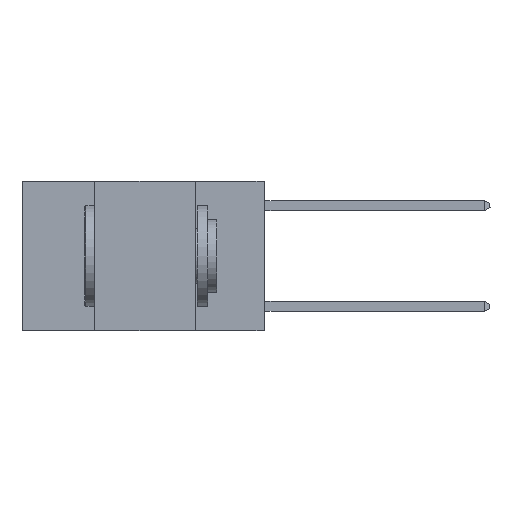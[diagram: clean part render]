
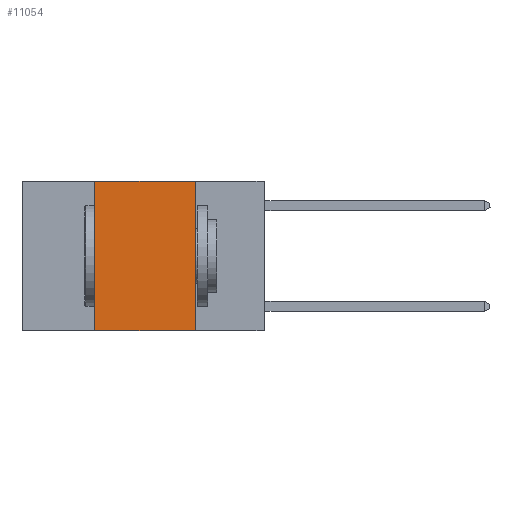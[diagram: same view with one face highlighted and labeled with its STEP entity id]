
A CAD part, left-side view. The second image highlights one B-rep face of the part: STEP entity #11054.
In plain terms, the highlighted planar face has unit normal (-1, 0, 0).
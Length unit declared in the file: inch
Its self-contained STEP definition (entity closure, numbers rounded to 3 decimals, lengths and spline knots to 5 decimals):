
#146 = CARTESIAN_POINT ( 'NONE',  ( 0., 0.6, -0.37 ) ) ;
#241 = VECTOR ( 'NONE', #4468, 39.37008 ) ;
#398 = AXIS2_PLACEMENT_3D ( 'NONE', #4768, #12748, #2808 ) ;
#622 = CARTESIAN_POINT ( 'NONE',  ( 0., 0.6, 0. ) ) ;
#764 = LINE ( 'NONE', #622, #5797 ) ;
#1096 = LINE ( 'NONE', #146, #2507 ) ;
#1280 = CARTESIAN_POINT ( 'NONE',  ( 0., 0.17, 0. ) ) ;
#1683 = CARTESIAN_POINT ( 'NONE',  ( 0., 0.17, 0. ) ) ;
#1985 = ORIENTED_EDGE ( 'NONE', *, *, #12948, .F. ) ;
#2211 = DIRECTION ( 'NONE',  ( 0., -1., 0. ) ) ;
#2241 = CARTESIAN_POINT ( 'NONE',  ( 0., 0.42, 0. ) ) ;
#2301 = CARTESIAN_POINT ( 'NONE',  ( 0., 0.42, 0. ) ) ;
#2507 = VECTOR ( 'NONE', #2211, 39.37008 ) ;
#2808 = DIRECTION ( 'NONE',  ( 0., 0., -1. ) ) ;
#3441 = LINE ( 'NONE', #2241, #241 ) ;
#3780 = CARTESIAN_POINT ( 'NONE',  ( 0., 0.42, -0.37 ) ) ;
#4468 = DIRECTION ( 'NONE',  ( 0., 0., 1. ) ) ;
#4728 = VERTEX_POINT ( 'NONE', #1280 ) ;
#4768 = CARTESIAN_POINT ( 'NONE',  ( 0., 0.6, 0. ) ) ;
#5736 = EDGE_CURVE ( 'NONE', #10228, #8686, #3441, .T. ) ;
#5797 = VECTOR ( 'NONE', #8819, 39.37008 ) ;
#6475 = ORIENTED_EDGE ( 'NONE', *, *, #5736, .F. ) ;
#6896 = FACE_OUTER_BOUND ( 'NONE', #11346, .T. ) ;
#8124 = EDGE_CURVE ( 'NONE', #8686, #4728, #764, .T. ) ;
#8580 = ORIENTED_EDGE ( 'NONE', *, *, #10670, .T. ) ;
#8686 = VERTEX_POINT ( 'NONE', #2301 ) ;
#8819 = DIRECTION ( 'NONE',  ( 0., -1., 0. ) ) ;
#9401 = ORIENTED_EDGE ( 'NONE', *, *, #8124, .F. ) ;
#10228 = VERTEX_POINT ( 'NONE', #3780 ) ;
#10670 = EDGE_CURVE ( 'NONE', #10228, #11645, #1096, .T. ) ;
#10779 = LINE ( 'NONE', #1683, #12958 ) ;
#10809 = CARTESIAN_POINT ( 'NONE',  ( 0., 0.17, -0.37 ) ) ;
#11054 = ADVANCED_FACE ( 'NONE', ( #6896 ), #13015, .F. ) ;
#11346 = EDGE_LOOP ( 'NONE', ( #1985, #9401, #6475, #8580 ) ) ;
#11645 = VERTEX_POINT ( 'NONE', #10809 ) ;
#12101 = DIRECTION ( 'NONE',  ( 0., 0., -1. ) ) ;
#12748 = DIRECTION ( 'NONE',  ( 1., 0., 0. ) ) ;
#12948 = EDGE_CURVE ( 'NONE', #4728, #11645, #10779, .T. ) ;
#12958 = VECTOR ( 'NONE', #12101, 39.37008 ) ;
#13015 = PLANE ( 'NONE',  #398 ) ;
